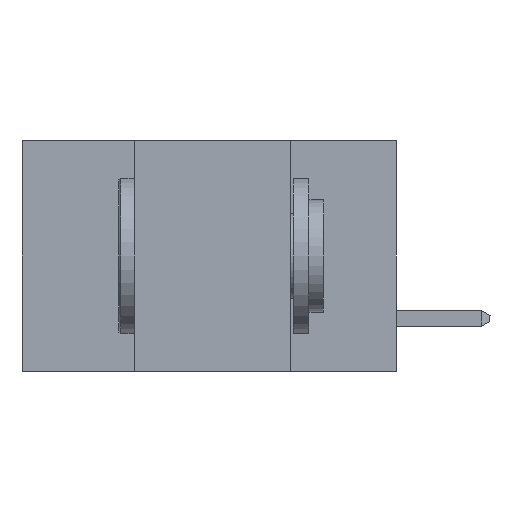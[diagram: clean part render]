
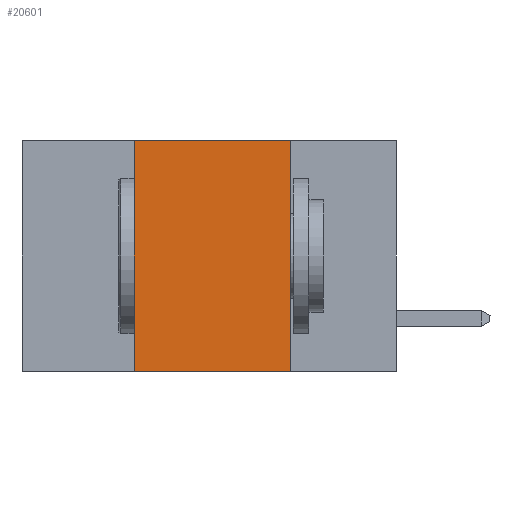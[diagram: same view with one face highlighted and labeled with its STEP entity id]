
A CAD part, left-side view. The second image highlights one B-rep face of the part: STEP entity #20601.
In plain terms, the highlighted planar face has unit normal (-1, 0, 0).
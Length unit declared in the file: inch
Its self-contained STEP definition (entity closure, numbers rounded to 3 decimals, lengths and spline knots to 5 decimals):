
#565 = VECTOR ( 'NONE', #13715, 39.37008 ) ;
#1856 = VECTOR ( 'NONE', #10275, 39.37008 ) ;
#2070 = DIRECTION ( 'NONE',  ( 0., -1., 0. ) ) ;
#2816 = EDGE_CURVE ( 'NONE', #12461, #19973, #9466, .T. ) ;
#3211 = ORIENTED_EDGE ( 'NONE', *, *, #20195, .F. ) ;
#4277 = DIRECTION ( 'NONE',  ( 1., 0., 0. ) ) ;
#4534 = CARTESIAN_POINT ( 'NONE',  ( 0., 0.42, -0.37 ) ) ;
#4625 = LINE ( 'NONE', #22580, #17933 ) ;
#5087 = PLANE ( 'NONE',  #7954 ) ;
#5282 = CARTESIAN_POINT ( 'NONE',  ( 0., 0.42, -0.37 ) ) ;
#5504 = ORIENTED_EDGE ( 'NONE', *, *, #2816, .F. ) ;
#5725 = CARTESIAN_POINT ( 'NONE',  ( 0., 0.17, -0.37 ) ) ;
#6434 = CARTESIAN_POINT ( 'NONE',  ( 0., 0.17, -0.37 ) ) ;
#7954 = AXIS2_PLACEMENT_3D ( 'NONE', #18875, #4277, #11804 ) ;
#8722 = ORIENTED_EDGE ( 'NONE', *, *, #21919, .T. ) ;
#9010 = EDGE_CURVE ( 'NONE', #19973, #12100, #22828, .T. ) ;
#9466 = LINE ( 'NONE', #18440, #11700 ) ;
#9936 = VERTEX_POINT ( 'NONE', #5282 ) ;
#10275 = DIRECTION ( 'NONE',  ( 0., 0., 1. ) ) ;
#11308 = CARTESIAN_POINT ( 'NONE',  ( 0., 0.42, 0. ) ) ;
#11700 = VECTOR ( 'NONE', #2070, 39.37008 ) ;
#11804 = DIRECTION ( 'NONE',  ( 0., 0., -1. ) ) ;
#12100 = VERTEX_POINT ( 'NONE', #5725 ) ;
#12461 = VERTEX_POINT ( 'NONE', #11308 ) ;
#13583 = FACE_OUTER_BOUND ( 'NONE', #23145, .T. ) ;
#13715 = DIRECTION ( 'NONE',  ( 0., 0., -1. ) ) ;
#17933 = VECTOR ( 'NONE', #19463, 39.37008 ) ;
#18440 = CARTESIAN_POINT ( 'NONE',  ( 0., 0.6, 0. ) ) ;
#18646 = ORIENTED_EDGE ( 'NONE', *, *, #9010, .F. ) ;
#18875 = CARTESIAN_POINT ( 'NONE',  ( 0., 0.6, 0. ) ) ;
#19463 = DIRECTION ( 'NONE',  ( 0., -1., 0. ) ) ;
#19653 = CARTESIAN_POINT ( 'NONE',  ( 0., 0.17, 0. ) ) ;
#19973 = VERTEX_POINT ( 'NONE', #19653 ) ;
#20195 = EDGE_CURVE ( 'NONE', #9936, #12461, #20926, .T. ) ;
#20601 = ADVANCED_FACE ( 'NONE', ( #13583 ), #5087, .F. ) ;
#20926 = LINE ( 'NONE', #4534, #1856 ) ;
#21919 = EDGE_CURVE ( 'NONE', #9936, #12100, #4625, .T. ) ;
#22580 = CARTESIAN_POINT ( 'NONE',  ( 0., 0.6, -0.37 ) ) ;
#22828 = LINE ( 'NONE', #6434, #565 ) ;
#23145 = EDGE_LOOP ( 'NONE', ( #18646, #5504, #3211, #8722 ) ) ;
